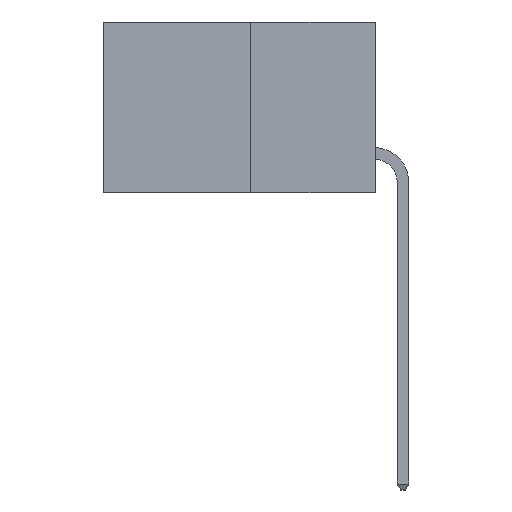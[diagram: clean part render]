
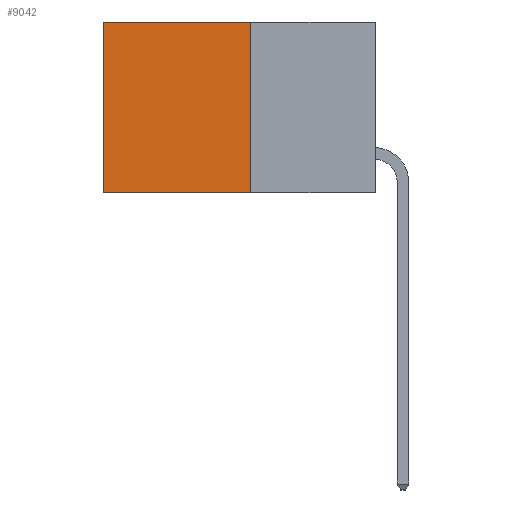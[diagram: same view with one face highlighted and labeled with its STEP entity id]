
A CAD part, left-side view. The second image highlights one B-rep face of the part: STEP entity #9042.
In plain terms, the highlighted planar face has unit normal (-1, 0, 0).
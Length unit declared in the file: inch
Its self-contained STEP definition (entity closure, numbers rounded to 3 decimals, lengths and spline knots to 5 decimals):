
#406 = VECTOR ( 'NONE', #427, 39.37008 ) ;
#427 = DIRECTION ( 'NONE',  ( 0., 1., 0. ) ) ;
#1168 = VERTEX_POINT ( 'NONE', #27330 ) ;
#1919 = CARTESIAN_POINT ( 'NONE',  ( 0.277, 0.27, -0.37 ) ) ;
#2336 = CARTESIAN_POINT ( 'NONE',  ( 0.277, 0.27, -0.37 ) ) ;
#4238 = DIRECTION ( 'NONE',  ( 0., 0., -1. ) ) ;
#4241 = AXIS2_PLACEMENT_3D ( 'NONE', #1919, #17998, #4238 ) ;
#4271 = VECTOR ( 'NONE', #17593, 39.37008 ) ;
#5082 = VERTEX_POINT ( 'NONE', #13707 ) ;
#6649 = VECTOR ( 'NONE', #18397, 39.37008 ) ;
#7383 = LINE ( 'NONE', #9214, #6649 ) ;
#7421 = FACE_OUTER_BOUND ( 'NONE', #15166, .T. ) ;
#8040 = VERTEX_POINT ( 'NONE', #28034 ) ;
#8586 = ORIENTED_EDGE ( 'NONE', *, *, #10944, .F. ) ;
#9042 = ADVANCED_FACE ( 'NONE', ( #7421 ), #11135, .F. ) ;
#9214 = CARTESIAN_POINT ( 'NONE',  ( 0.277, 0.59, -0.37 ) ) ;
#10634 = ORIENTED_EDGE ( 'NONE', *, *, #27781, .T. ) ;
#10944 = EDGE_CURVE ( 'NONE', #8040, #11756, #23902, .T. ) ;
#11135 = PLANE ( 'NONE',  #4241 ) ;
#11175 = ORIENTED_EDGE ( 'NONE', *, *, #21666, .T. ) ;
#11546 = DIRECTION ( 'NONE',  ( 0., 0., -1. ) ) ;
#11756 = VERTEX_POINT ( 'NONE', #17071 ) ;
#13426 = EDGE_CURVE ( 'NONE', #5082, #8040, #19947, .T. ) ;
#13707 = CARTESIAN_POINT ( 'NONE',  ( 0.277, 0.27, 0. ) ) ;
#13929 = VECTOR ( 'NONE', #11546, 39.37008 ) ;
#14228 = CARTESIAN_POINT ( 'NONE',  ( 0.277, 0.27, -0.37 ) ) ;
#15166 = EDGE_LOOP ( 'NONE', ( #11175, #8586, #15326, #10634 ) ) ;
#15290 = CARTESIAN_POINT ( 'NONE',  ( 0.277, 0.27, 0. ) ) ;
#15326 = ORIENTED_EDGE ( 'NONE', *, *, #13426, .F. ) ;
#17071 = CARTESIAN_POINT ( 'NONE',  ( 0.277, 0.59, -0.37 ) ) ;
#17593 = DIRECTION ( 'NONE',  ( 0., 1., 0. ) ) ;
#17998 = DIRECTION ( 'NONE',  ( 1., 0., 0. ) ) ;
#18397 = DIRECTION ( 'NONE',  ( 0., 0., -1. ) ) ;
#19947 = LINE ( 'NONE', #2336, #13929 ) ;
#21666 = EDGE_CURVE ( 'NONE', #1168, #11756, #7383, .T. ) ;
#22425 = LINE ( 'NONE', #15290, #4271 ) ;
#23902 = LINE ( 'NONE', #14228, #406 ) ;
#27330 = CARTESIAN_POINT ( 'NONE',  ( 0.277, 0.59, 0. ) ) ;
#27781 = EDGE_CURVE ( 'NONE', #5082, #1168, #22425, .T. ) ;
#28034 = CARTESIAN_POINT ( 'NONE',  ( 0.277, 0.27, -0.37 ) ) ;
